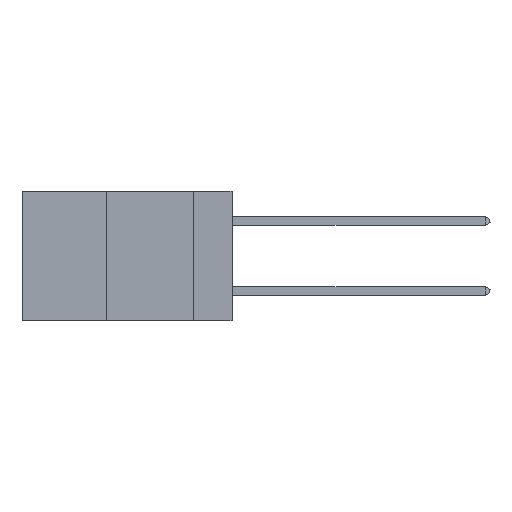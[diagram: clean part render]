
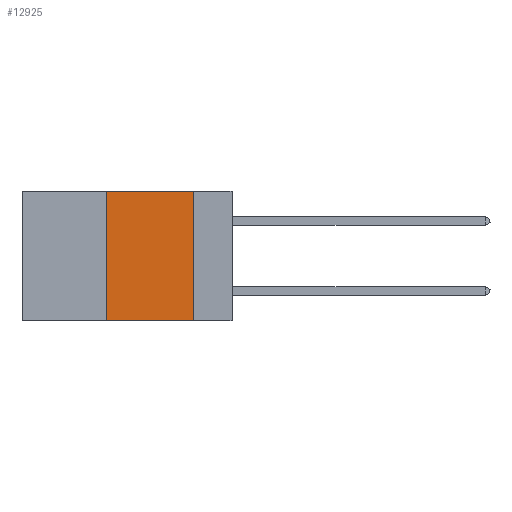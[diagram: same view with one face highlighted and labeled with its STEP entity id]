
A CAD part, left-side view. The second image highlights one B-rep face of the part: STEP entity #12925.
In plain terms, the highlighted planar face has unit normal (-1, 0, 0).
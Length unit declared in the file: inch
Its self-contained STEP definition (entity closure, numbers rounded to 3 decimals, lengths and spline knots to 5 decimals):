
#44 = VECTOR ( 'NONE', #469, 39.37008 ) ;
#469 = DIRECTION ( 'NONE',  ( 0., 0., -1. ) ) ;
#1319 = PLANE ( 'NONE',  #5456 ) ;
#1909 = CARTESIAN_POINT ( 'NONE',  ( 0., 0.6, -0.37 ) ) ;
#2863 = CARTESIAN_POINT ( 'NONE',  ( 0., 0.36, 0. ) ) ;
#4175 = LINE ( 'NONE', #1909, #13603 ) ;
#4384 = VERTEX_POINT ( 'NONE', #2863 ) ;
#4542 = FACE_OUTER_BOUND ( 'NONE', #21457, .T. ) ;
#5439 = DIRECTION ( 'NONE',  ( 1., 0., 0. ) ) ;
#5456 = AXIS2_PLACEMENT_3D ( 'NONE', #9454, #5439, #19304 ) ;
#7148 = EDGE_CURVE ( 'NONE', #4384, #20690, #19161, .T. ) ;
#7972 = EDGE_CURVE ( 'NONE', #21677, #25265, #4175, .T. ) ;
#8722 = ORIENTED_EDGE ( 'NONE', *, *, #12039, .F. ) ;
#9322 = EDGE_CURVE ( 'NONE', #21677, #4384, #9790, .T. ) ;
#9454 = CARTESIAN_POINT ( 'NONE',  ( 0., 0.6, 0. ) ) ;
#9790 = LINE ( 'NONE', #20336, #19593 ) ;
#12039 = EDGE_CURVE ( 'NONE', #20690, #25265, #20683, .T. ) ;
#12185 = VECTOR ( 'NONE', #17081, 39.37008 ) ;
#12925 = ADVANCED_FACE ( 'NONE', ( #4542 ), #1319, .F. ) ;
#13603 = VECTOR ( 'NONE', #14029, 39.37008 ) ;
#14029 = DIRECTION ( 'NONE',  ( 0., -1., 0. ) ) ;
#16568 = CARTESIAN_POINT ( 'NONE',  ( 0., 0.11, 0. ) ) ;
#17081 = DIRECTION ( 'NONE',  ( 0., -1., 0. ) ) ;
#17358 = ORIENTED_EDGE ( 'NONE', *, *, #7972, .T. ) ;
#18857 = ORIENTED_EDGE ( 'NONE', *, *, #7148, .F. ) ;
#19161 = LINE ( 'NONE', #22987, #12185 ) ;
#19304 = DIRECTION ( 'NONE',  ( 0., 0., -1. ) ) ;
#19593 = VECTOR ( 'NONE', #22325, 39.37008 ) ;
#20336 = CARTESIAN_POINT ( 'NONE',  ( 0., 0.36, 0. ) ) ;
#20683 = LINE ( 'NONE', #16568, #44 ) ;
#20690 = VERTEX_POINT ( 'NONE', #22984 ) ;
#21457 = EDGE_LOOP ( 'NONE', ( #8722, #18857, #24087, #17358 ) ) ;
#21677 = VERTEX_POINT ( 'NONE', #25552 ) ;
#22325 = DIRECTION ( 'NONE',  ( 0., 0., 1. ) ) ;
#22984 = CARTESIAN_POINT ( 'NONE',  ( 0., 0.11, 0. ) ) ;
#22987 = CARTESIAN_POINT ( 'NONE',  ( 0., 0.6, 0. ) ) ;
#24087 = ORIENTED_EDGE ( 'NONE', *, *, #9322, .F. ) ;
#24240 = CARTESIAN_POINT ( 'NONE',  ( 0., 0.11, -0.37 ) ) ;
#25265 = VERTEX_POINT ( 'NONE', #24240 ) ;
#25552 = CARTESIAN_POINT ( 'NONE',  ( 0., 0.36, -0.37 ) ) ;
